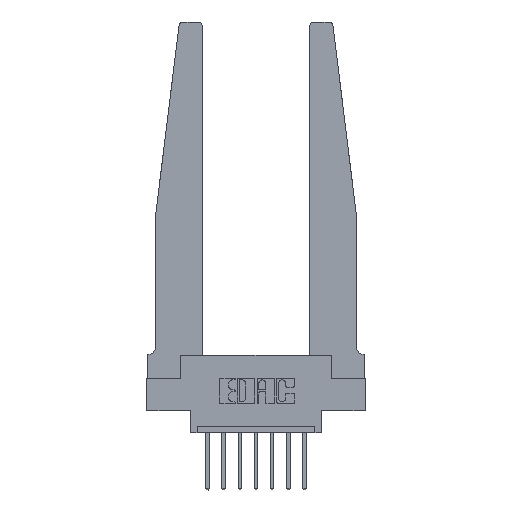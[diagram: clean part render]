
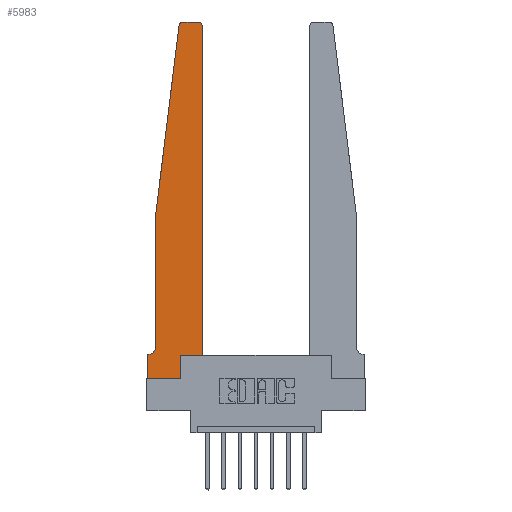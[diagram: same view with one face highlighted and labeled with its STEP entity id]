
A CAD part, top view. The second image highlights one B-rep face of the part: STEP entity #5983.
In plain terms, the highlighted planar face has unit normal (0, 0, 1).
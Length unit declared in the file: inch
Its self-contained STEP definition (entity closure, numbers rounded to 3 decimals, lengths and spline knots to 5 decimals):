
#79 = EDGE_CURVE ( 'NONE', #119, #1371, #6853, .T. ) ;
#100 = VECTOR ( 'NONE', #4802, 39.37008 ) ;
#119 = VERTEX_POINT ( 'NONE', #8284 ) ;
#145 = EDGE_CURVE ( 'NONE', #11863, #305, #1987, .T. ) ;
#258 = DIRECTION ( 'NONE',  ( 1., 0., 0. ) ) ;
#305 = VERTEX_POINT ( 'NONE', #4068 ) ;
#884 = FACE_OUTER_BOUND ( 'NONE', #13790, .T. ) ;
#973 = DIRECTION ( 'NONE',  ( -0.122, -0.992, 0. ) ) ;
#1006 = VERTEX_POINT ( 'NONE', #5936 ) ;
#1097 = PLANE ( 'NONE',  #9418 ) ;
#1371 = VERTEX_POINT ( 'NONE', #12953 ) ;
#1803 = DIRECTION ( 'NONE',  ( -1., 0., 0. ) ) ;
#1908 = DIRECTION ( 'NONE',  ( 1., 0., 0. ) ) ;
#1987 = CIRCLE ( 'NONE', #13882, 0.03 ) ;
#2279 = VECTOR ( 'NONE', #13336, 39.37008 ) ;
#2313 = LINE ( 'NONE', #11963, #3609 ) ;
#2421 = DIRECTION ( 'NONE',  ( 0., -1., 0. ) ) ;
#2450 = VERTEX_POINT ( 'NONE', #10264 ) ;
#2570 = CARTESIAN_POINT ( 'NONE',  ( 0.065, 0.1875, 0.37 ) ) ;
#2716 = VECTOR ( 'NONE', #9889, 39.37008 ) ;
#2878 = VERTEX_POINT ( 'NONE', #3098 ) ;
#2951 = CARTESIAN_POINT ( 'NONE',  ( 0.015, 0.2375, 0.37 ) ) ;
#3098 = CARTESIAN_POINT ( 'NONE',  ( 0.425, 2.72, 0.37 ) ) ;
#3193 = AXIS2_PLACEMENT_3D ( 'NONE', #2951, #14245, #1803 ) ;
#3198 = DIRECTION ( 'NONE',  ( 0., 0., 1. ) ) ;
#3207 = LINE ( 'NONE', #10908, #10029 ) ;
#3403 = ORIENTED_EDGE ( 'NONE', *, *, #8396, .T. ) ;
#3609 = VECTOR ( 'NONE', #1908, 39.37008 ) ;
#3815 = VECTOR ( 'NONE', #8635, 39.37008 ) ;
#4068 = CARTESIAN_POINT ( 'NONE',  ( 0.24675, 2.72367, 0.37 ) ) ;
#4347 = AXIS2_PLACEMENT_3D ( 'NONE', #11749, #9517, #6131 ) ;
#4503 = CARTESIAN_POINT ( 'NONE',  ( 0.065, 1.25, 0.37 ) ) ;
#4664 = CARTESIAN_POINT ( 'NONE',  ( 0.25, 2.75, 0.37 ) ) ;
#4802 = DIRECTION ( 'NONE',  ( 0., 1., 0. ) ) ;
#4966 = ORIENTED_EDGE ( 'NONE', *, *, #7228, .T. ) ;
#5077 = VERTEX_POINT ( 'NONE', #11272 ) ;
#5190 = ORIENTED_EDGE ( 'NONE', *, *, #12863, .T. ) ;
#5535 = CARTESIAN_POINT ( 'NONE',  ( 0.27653, 2.72, 0.37 ) ) ;
#5641 = VECTOR ( 'NONE', #10559, 39.37008 ) ;
#5702 = ORIENTED_EDGE ( 'NONE', *, *, #8965, .T. ) ;
#5796 = VERTEX_POINT ( 'NONE', #8128 ) ;
#5936 = CARTESIAN_POINT ( 'NONE',  ( 0.2605, 0.18, 0.37 ) ) ;
#5983 = ADVANCED_FACE ( 'NONE', ( #884 ), #1097, .T. ) ;
#6131 = DIRECTION ( 'NONE',  ( 1., 0., 0. ) ) ;
#6268 = VERTEX_POINT ( 'NONE', #10922 ) ;
#6345 = EDGE_CURVE ( 'NONE', #5796, #11863, #10116, .T. ) ;
#6746 = LINE ( 'NONE', #10218, #2279 ) ;
#6853 = LINE ( 'NONE', #7933, #10356 ) ;
#7038 = VECTOR ( 'NONE', #7353, 39.37008 ) ;
#7228 = EDGE_CURVE ( 'NONE', #6268, #2878, #6746, .T. ) ;
#7300 = ORIENTED_EDGE ( 'NONE', *, *, #6345, .T. ) ;
#7353 = DIRECTION ( 'NONE',  ( 1., 0., 0. ) ) ;
#7409 = EDGE_CURVE ( 'NONE', #5077, #11793, #9407, .T. ) ;
#7933 = CARTESIAN_POINT ( 'NONE',  ( 0., 0., 0.37 ) ) ;
#8006 = LINE ( 'NONE', #11354, #100 ) ;
#8128 = CARTESIAN_POINT ( 'NONE',  ( 0.395, 2.75, 0.37 ) ) ;
#8129 = ORIENTED_EDGE ( 'NONE', *, *, #7409, .T. ) ;
#8284 = CARTESIAN_POINT ( 'NONE',  ( 0., 0.1875, 0.37 ) ) ;
#8396 = EDGE_CURVE ( 'NONE', #1006, #6268, #2313, .T. ) ;
#8429 = LINE ( 'NONE', #13211, #7038 ) ;
#8635 = DIRECTION ( 'NONE',  ( 0., -1., 0. ) ) ;
#8698 = EDGE_CURVE ( 'NONE', #13716, #5077, #9850, .T. ) ;
#8965 = EDGE_CURVE ( 'NONE', #2878, #5796, #13198, .T. ) ;
#9407 = CIRCLE ( 'NONE', #3193, 0.05 ) ;
#9418 = AXIS2_PLACEMENT_3D ( 'NONE', #10220, #11265, #258 ) ;
#9517 = DIRECTION ( 'NONE',  ( 0., 0., 1. ) ) ;
#9850 = LINE ( 'NONE', #11035, #3815 ) ;
#9889 = DIRECTION ( 'NONE',  ( -1., 0., 0. ) ) ;
#10029 = VECTOR ( 'NONE', #973, 39.37008 ) ;
#10116 = LINE ( 'NONE', #4664, #2716 ) ;
#10218 = CARTESIAN_POINT ( 'NONE',  ( 0.425, 0.18, 0.37 ) ) ;
#10220 = CARTESIAN_POINT ( 'NONE',  ( 0., 0.1875, 0.37 ) ) ;
#10264 = CARTESIAN_POINT ( 'NONE',  ( 0.2605, 0., 0.37 ) ) ;
#10267 = LINE ( 'NONE', #2570, #5641 ) ;
#10356 = VECTOR ( 'NONE', #2421, 39.37008 ) ;
#10559 = DIRECTION ( 'NONE',  ( -1., 0., 0. ) ) ;
#10843 = EDGE_CURVE ( 'NONE', #305, #13716, #3207, .T. ) ;
#10895 = DIRECTION ( 'NONE',  ( 1., 0., 0. ) ) ;
#10908 = CARTESIAN_POINT ( 'NONE',  ( 0.065, 1.25, 0.37 ) ) ;
#10922 = CARTESIAN_POINT ( 'NONE',  ( 0.425, 0.18, 0.37 ) ) ;
#11035 = CARTESIAN_POINT ( 'NONE',  ( 0.065, 1.25, 0.37 ) ) ;
#11241 = ORIENTED_EDGE ( 'NONE', *, *, #10843, .T. ) ;
#11265 = DIRECTION ( 'NONE',  ( 0., 0., 1. ) ) ;
#11272 = CARTESIAN_POINT ( 'NONE',  ( 0.065, 0.2375, 0.37 ) ) ;
#11354 = CARTESIAN_POINT ( 'NONE',  ( 0.2605, 0.18, 0.37 ) ) ;
#11749 = CARTESIAN_POINT ( 'NONE',  ( 0.395, 2.72, 0.37 ) ) ;
#11793 = VERTEX_POINT ( 'NONE', #13551 ) ;
#11863 = VERTEX_POINT ( 'NONE', #14108 ) ;
#11963 = CARTESIAN_POINT ( 'NONE',  ( 0.425, 0.18, 0.37 ) ) ;
#12031 = ORIENTED_EDGE ( 'NONE', *, *, #79, .T. ) ;
#12420 = EDGE_CURVE ( 'NONE', #2450, #1006, #8006, .T. ) ;
#12804 = EDGE_CURVE ( 'NONE', #11793, #119, #10267, .T. ) ;
#12863 = EDGE_CURVE ( 'NONE', #1371, #2450, #8429, .T. ) ;
#12953 = CARTESIAN_POINT ( 'NONE',  ( 0., 0., 0.37 ) ) ;
#13198 = CIRCLE ( 'NONE', #4347, 0.03 ) ;
#13211 = CARTESIAN_POINT ( 'NONE',  ( 0., 0., 0.37 ) ) ;
#13336 = DIRECTION ( 'NONE',  ( 0., 1., 0. ) ) ;
#13340 = ORIENTED_EDGE ( 'NONE', *, *, #145, .T. ) ;
#13551 = CARTESIAN_POINT ( 'NONE',  ( 0.015, 0.1875, 0.37 ) ) ;
#13716 = VERTEX_POINT ( 'NONE', #4503 ) ;
#13790 = EDGE_LOOP ( 'NONE', ( #7300, #13340, #11241, #13945, #8129, #14196, #12031, #5190, #13904, #3403, #4966, #5702 ) ) ;
#13882 = AXIS2_PLACEMENT_3D ( 'NONE', #5535, #3198, #10895 ) ;
#13904 = ORIENTED_EDGE ( 'NONE', *, *, #12420, .T. ) ;
#13945 = ORIENTED_EDGE ( 'NONE', *, *, #8698, .T. ) ;
#14108 = CARTESIAN_POINT ( 'NONE',  ( 0.27653, 2.75, 0.37 ) ) ;
#14196 = ORIENTED_EDGE ( 'NONE', *, *, #12804, .T. ) ;
#14245 = DIRECTION ( 'NONE',  ( 0., 0., -1. ) ) ;
